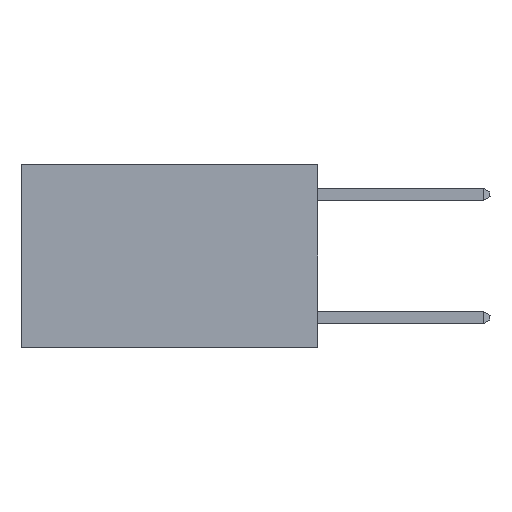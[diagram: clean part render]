
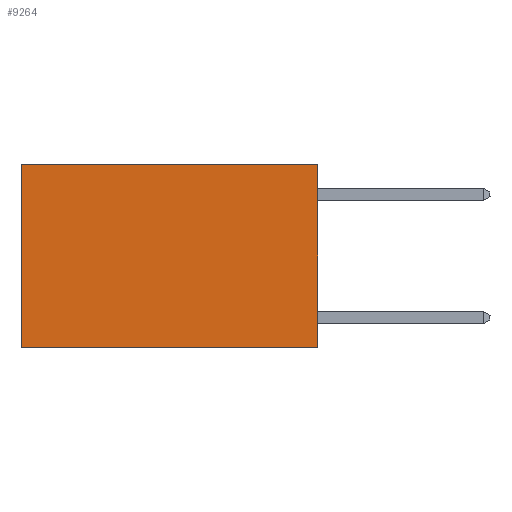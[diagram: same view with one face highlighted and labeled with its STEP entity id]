
A CAD part, left-side view. The second image highlights one B-rep face of the part: STEP entity #9264.
In plain terms, the highlighted planar face has unit normal (-1, 0, 0).
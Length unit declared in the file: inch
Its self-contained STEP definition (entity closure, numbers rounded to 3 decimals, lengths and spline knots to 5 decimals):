
#25 = VERTEX_POINT ( 'NONE', #6915 ) ;
#200 = ORIENTED_EDGE ( 'NONE', *, *, #7539, .F. ) ;
#222 = VECTOR ( 'NONE', #4391, 39.37008 ) ;
#612 = LINE ( 'NONE', #7932, #10143 ) ;
#1257 = DIRECTION ( 'NONE',  ( 1., 0., 0. ) ) ;
#2137 = EDGE_CURVE ( 'NONE', #3266, #25, #6842, .T. ) ;
#2469 = LINE ( 'NONE', #9179, #5410 ) ;
#2568 = ORIENTED_EDGE ( 'NONE', *, *, #2137, .T. ) ;
#2974 = CARTESIAN_POINT ( 'NONE',  ( 0.2625, 0.6, 0. ) ) ;
#3051 = EDGE_CURVE ( 'NONE', #8051, #3266, #2469, .T. ) ;
#3266 = VERTEX_POINT ( 'NONE', #5501 ) ;
#3885 = DIRECTION ( 'NONE',  ( 0., 0., -1. ) ) ;
#3966 = EDGE_LOOP ( 'NONE', ( #2568, #6954, #200, #8542 ) ) ;
#4391 = DIRECTION ( 'NONE',  ( 0., 0., -1. ) ) ;
#4557 = CARTESIAN_POINT ( 'NONE',  ( 0.2625, 0., 0. ) ) ;
#4569 = CARTESIAN_POINT ( 'NONE',  ( 0.2625, 0., -0.37 ) ) ;
#4827 = CARTESIAN_POINT ( 'NONE',  ( 0.2625, 0., -0.37 ) ) ;
#5410 = VECTOR ( 'NONE', #7563, 39.37008 ) ;
#5474 = CARTESIAN_POINT ( 'NONE',  ( 0.2625, 0., 0. ) ) ;
#5501 = CARTESIAN_POINT ( 'NONE',  ( 0.2625, 0.6, 0. ) ) ;
#5517 = FACE_OUTER_BOUND ( 'NONE', #3966, .T. ) ;
#5818 = DIRECTION ( 'NONE',  ( 0., 1., 0. ) ) ;
#6244 = EDGE_CURVE ( 'NONE', #7600, #25, #9793, .T. ) ;
#6842 = LINE ( 'NONE', #2974, #222 ) ;
#6915 = CARTESIAN_POINT ( 'NONE',  ( 0.2625, 0.6, -0.37 ) ) ;
#6954 = ORIENTED_EDGE ( 'NONE', *, *, #6244, .F. ) ;
#7539 = EDGE_CURVE ( 'NONE', #8051, #7600, #612, .T. ) ;
#7563 = DIRECTION ( 'NONE',  ( 0., 1., 0. ) ) ;
#7600 = VERTEX_POINT ( 'NONE', #4569 ) ;
#7932 = CARTESIAN_POINT ( 'NONE',  ( 0.2625, 0., 0. ) ) ;
#8051 = VERTEX_POINT ( 'NONE', #4557 ) ;
#8542 = ORIENTED_EDGE ( 'NONE', *, *, #3051, .T. ) ;
#8794 = AXIS2_PLACEMENT_3D ( 'NONE', #5474, #1257, #3885 ) ;
#9179 = CARTESIAN_POINT ( 'NONE',  ( 0.2625, 0., 0. ) ) ;
#9264 = ADVANCED_FACE ( 'NONE', ( #5517 ), #9627, .F. ) ;
#9627 = PLANE ( 'NONE',  #8794 ) ;
#9681 = VECTOR ( 'NONE', #5818, 39.37008 ) ;
#9793 = LINE ( 'NONE', #4827, #9681 ) ;
#10143 = VECTOR ( 'NONE', #10327, 39.37008 ) ;
#10327 = DIRECTION ( 'NONE',  ( 0., 0., -1. ) ) ;
